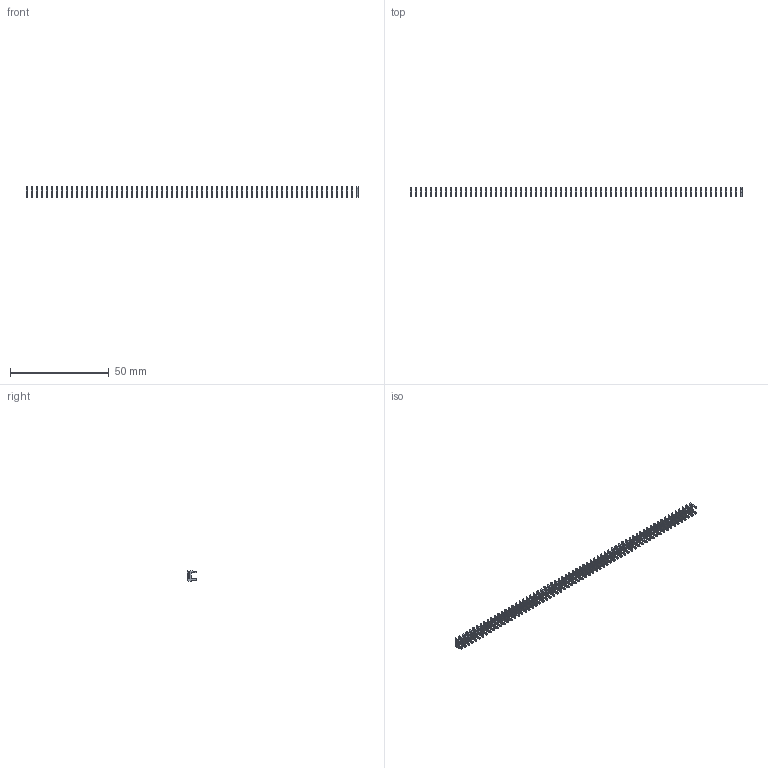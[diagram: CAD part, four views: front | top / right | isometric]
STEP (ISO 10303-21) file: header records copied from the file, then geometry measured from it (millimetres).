
FILE_DESCRIPTION (( 'STEP AP203' ), '1' );
FILE_NAME ('105-067-208-100.STEP', '2020-04-08T01:01:05', ( '' ), ( '' ), 'SwSTEP 2.0', 'SolidWorks 2016', '' );
FILE_SCHEMA (( 'CONFIG_CONTROL_DESIGN' ));
Length unit declared in the file: inch
Products named in the file (2): 100-290-001_100-290-208; 105-067-208-100
Assembly tree (67 placements, depth 2):
  105-067-208-100
    100-290-001_100-290-208  x67
Bounding box: 168.15 x 4.83 x 5.17 mm (x, y, z)
Volume: 461 mm3; surface area: 2847.2 mm2
Topology: 67 solids, 67 shells, 1675 faces, 4623 edges, 3082 vertices
Faces by surface type: plane 1474, cylinder 201
Entity records: 3101 total; most frequent: DIRECTION 265, CARTESIAN_POINT 210, LOCAL_TIME 144, DATE_AND_TIME 144, COORDINATED_UNIVERSAL_TIME_OFFSET 144, CALENDAR_DATE 144, ORIENTED_EDGE 138, AXIS2_PLACEMENT_3D 101
